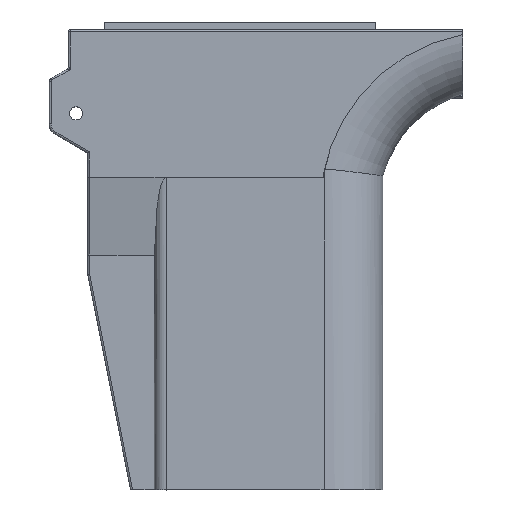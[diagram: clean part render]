
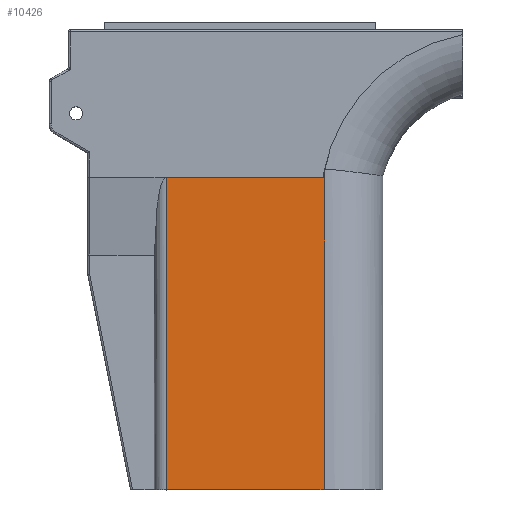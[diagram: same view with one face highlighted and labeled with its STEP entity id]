
A CAD part, top view. The second image highlights one B-rep face of the part: STEP entity #10426.
In plain terms, the highlighted planar face has unit normal (0, 0, 1).
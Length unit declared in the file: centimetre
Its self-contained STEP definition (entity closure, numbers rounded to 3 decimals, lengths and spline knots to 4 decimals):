
#308=PLANE($,#11142);
#673=FACE_OUTER_BOUND($,#1329,.T.);
#1329=EDGE_LOOP($,(#7283,#7284,#7285,#7286,#7287,#7288,#7289,#7290));
#2036=CIRCLE($,#11143,4.4939);
#2386=LINE($,#15388,#3412);
#2443=LINE($,#15621,#3469);
#2444=LINE($,#15623,#3470);
#2449=LINE($,#15640,#3475);
#2475=LINE($,#15765,#3501);
#2476=LINE($,#15766,#3502);
#2477=LINE($,#15769,#3503);
#3412=VECTOR($,#12153,8.2388);
#3469=VECTOR($,#12300,0.18);
#3470=VECTOR($,#12301,3.9);
#3475=VECTOR($,#12316,8.0449);
#3501=VECTOR($,#12416,4.0366);
#3502=VECTOR($,#12417,0.0001);
#3503=VECTOR($,#12420,0.0062);
#4517=VERTEX_POINT($,#15382);
#4518=VERTEX_POINT($,#15387);
#4598=VERTEX_POINT($,#15620);
#4599=VERTEX_POINT($,#15622);
#4606=VERTEX_POINT($,#15637);
#4636=VERTEX_POINT($,#15763);
#4637=VERTEX_POINT($,#15764);
#4638=VERTEX_POINT($,#15767);
#5478=EDGE_CURVE($,#4517,#4518,#2386,.T.);
#5573=EDGE_CURVE($,#4598,#4518,#2443,.F.);
#5574=EDGE_CURVE($,#4599,#4598,#2444,.F.);
#5583=EDGE_CURVE($,#4599,#4606,#2449,.T.);
#5631=EDGE_CURVE($,#4636,#4637,#2475,.T.);
#5632=EDGE_CURVE($,#4606,#4636,#2476,.F.);
#5633=EDGE_CURVE($,#4638,#4517,#2036,.T.);
#5634=EDGE_CURVE($,#4637,#4638,#2477,.T.);
#7283=ORIENTED_EDGE($,*,*,#5631,.F.);
#7284=ORIENTED_EDGE($,*,*,#5632,.F.);
#7285=ORIENTED_EDGE($,*,*,#5583,.F.);
#7286=ORIENTED_EDGE($,*,*,#5574,.T.);
#7287=ORIENTED_EDGE($,*,*,#5573,.T.);
#7288=ORIENTED_EDGE($,*,*,#5478,.F.);
#7289=ORIENTED_EDGE($,*,*,#5633,.F.);
#7290=ORIENTED_EDGE($,*,*,#5634,.F.);
#10426=ADVANCED_FACE($,(#673),#308,.F.);
#11142=AXIS2_PLACEMENT_3D($,#15762,#12414,#12415);
#11143=AXIS2_PLACEMENT_3D($,#15768,#12418,#12419);
#12153=DIRECTION($,(0.,-1.,0.));
#12300=DIRECTION($,(-1.,0.,0.));
#12301=DIRECTION($,(-1.,0.,0.));
#12316=DIRECTION($,(0.,1.,0.));
#12414=DIRECTION('center_axis',(0.,0.,
-1.));
#12415=DIRECTION('ref_axis',(0.,-1.,0.));
#12416=DIRECTION($,(1.,0.,0.));
#12417=DIRECTION($,(0.,-0.989,-0.148));
#12418=DIRECTION('center_axis',(0.,0.,
-1.));
#12419=DIRECTION('ref_axis',(-1.,0.,0.));
#12420=DIRECTION($,(1.,0.,0.));
#15382=CARTESIAN_POINT('',(-2.3936,-4.4352,2.));
#15387=CARTESIAN_POINT('',(-2.3936,-12.674,2.));
#15388=CARTESIAN_POINT($,(-2.3936,-12.674,2.));
#15620=CARTESIAN_POINT('',(-2.5736,-12.674,2.));
#15621=CARTESIAN_POINT($,(-4.4752,-12.674,2.));
#15622=CARTESIAN_POINT('',(-6.4736,-12.674,2.));
#15623=CARTESIAN_POINT($,(-4.4752,-12.674,2.));
#15637=CARTESIAN_POINT('',(-6.4736,-4.6291,2.));
#15640=CARTESIAN_POINT($,(-6.4736,-12.4244,2.));
#15762=CARTESIAN_POINT('Origin',(-4.4736,-12.4244,2.));
#15763=CARTESIAN_POINT('',(-6.4736,-4.629,2.));
#15764=CARTESIAN_POINT('',(-2.4371,-4.629,2.));
#15765=CARTESIAN_POINT($,(-2.964,-4.629,2.));
#15766=CARTESIAN_POINT($,(-6.4736,-5.7518,1.8316));
#15767=CARTESIAN_POINT('',(-2.4308,-4.629,2.));
#15768=CARTESIAN_POINT('Origin',(2.,-5.379,2.));
#15769=CARTESIAN_POINT($,(-2.964,-4.629,2.));
